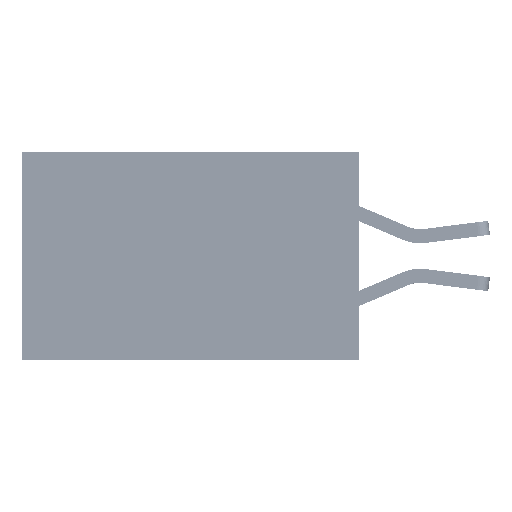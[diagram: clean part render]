
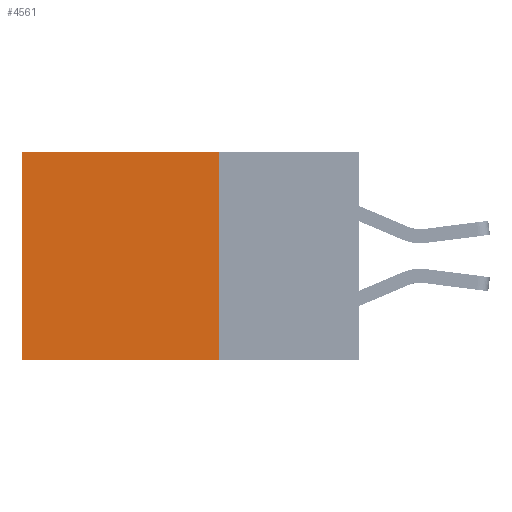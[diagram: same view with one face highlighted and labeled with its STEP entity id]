
A CAD part, left-side view. The second image highlights one B-rep face of the part: STEP entity #4561.
In plain terms, the highlighted planar face has unit normal (-1, 0, 0).
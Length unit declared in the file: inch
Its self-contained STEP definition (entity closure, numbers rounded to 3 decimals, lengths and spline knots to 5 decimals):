
#125 = ORIENTED_EDGE ( 'NONE', *, *, #27070, .T. ) ;
#157 = EDGE_CURVE ( 'NONE', #21451, #38829, #9441, .T. ) ;
#1656 = DIRECTION ( 'NONE',  ( 0., 1., 0. ) ) ;
#2776 = CARTESIAN_POINT ( 'NONE',  ( 0.2875, 0.6, 0. ) ) ;
#4561 = ADVANCED_FACE ( 'NONE', ( #4566 ), #17479, .F. ) ;
#4566 = FACE_OUTER_BOUND ( 'NONE', #24046, .T. ) ;
#5230 = VECTOR ( 'NONE', #40271, 39.37008 ) ;
#5602 = DIRECTION ( 'NONE',  ( 0., 0., -1. ) ) ;
#7262 = DIRECTION ( 'NONE',  ( 0., 0., -1. ) ) ;
#7613 = ORIENTED_EDGE ( 'NONE', *, *, #35378, .F. ) ;
#8984 = LINE ( 'NONE', #2776, #5230 ) ;
#9441 = LINE ( 'NONE', #25101, #25013 ) ;
#10448 = DIRECTION ( 'NONE',  ( 1., 0., 0. ) ) ;
#10737 = CARTESIAN_POINT ( 'NONE',  ( 0.2875, 0.25, 0. ) ) ;
#13602 = VERTEX_POINT ( 'NONE', #25141 ) ;
#13673 = AXIS2_PLACEMENT_3D ( 'NONE', #10737, #10448, #7262 ) ;
#14142 = VERTEX_POINT ( 'NONE', #27669 ) ;
#15089 = CARTESIAN_POINT ( 'NONE',  ( 0.2875, 0.25, 0. ) ) ;
#17479 = PLANE ( 'NONE',  #13673 ) ;
#21451 = VERTEX_POINT ( 'NONE', #37493 ) ;
#22181 = CARTESIAN_POINT ( 'NONE',  ( 0.2875, 0.25, 0. ) ) ;
#24046 = EDGE_LOOP ( 'NONE', ( #125, #40324, #7613, #24417 ) ) ;
#24087 = LINE ( 'NONE', #22181, #38584 ) ;
#24417 = ORIENTED_EDGE ( 'NONE', *, *, #33904, .T. ) ;
#25013 = VECTOR ( 'NONE', #28579, 39.37008 ) ;
#25101 = CARTESIAN_POINT ( 'NONE',  ( 0.2875, 0.25, -0.37 ) ) ;
#25141 = CARTESIAN_POINT ( 'NONE',  ( 0.2875, 0.25, 0. ) ) ;
#27070 = EDGE_CURVE ( 'NONE', #14142, #38829, #8984, .T. ) ;
#27669 = CARTESIAN_POINT ( 'NONE',  ( 0.2875, 0.6, 0. ) ) ;
#28579 = DIRECTION ( 'NONE',  ( 0., 1., 0. ) ) ;
#29318 = VECTOR ( 'NONE', #5602, 39.37008 ) ;
#31969 = LINE ( 'NONE', #15089, #29318 ) ;
#33904 = EDGE_CURVE ( 'NONE', #13602, #14142, #24087, .T. ) ;
#35378 = EDGE_CURVE ( 'NONE', #13602, #21451, #31969, .T. ) ;
#37493 = CARTESIAN_POINT ( 'NONE',  ( 0.2875, 0.25, -0.37 ) ) ;
#38584 = VECTOR ( 'NONE', #1656, 39.37008 ) ;
#38829 = VERTEX_POINT ( 'NONE', #42682 ) ;
#40271 = DIRECTION ( 'NONE',  ( 0., 0., -1. ) ) ;
#40324 = ORIENTED_EDGE ( 'NONE', *, *, #157, .F. ) ;
#42682 = CARTESIAN_POINT ( 'NONE',  ( 0.2875, 0.6, -0.37 ) ) ;
